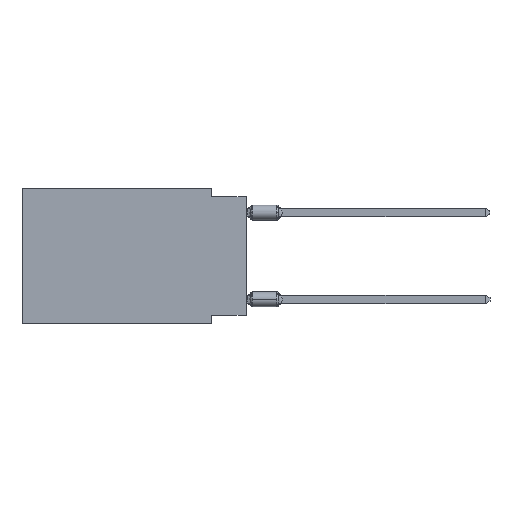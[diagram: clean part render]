
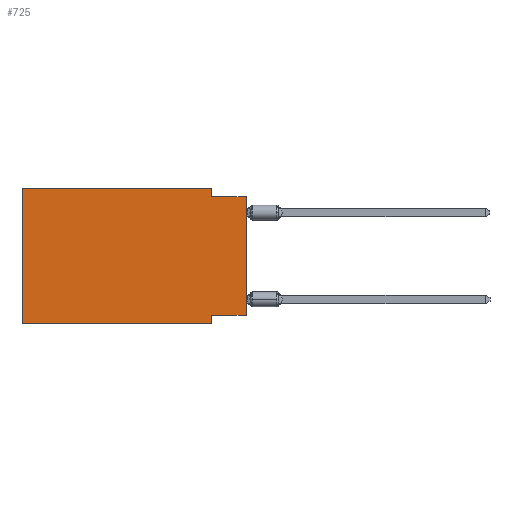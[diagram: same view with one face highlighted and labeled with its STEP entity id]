
A CAD part, left-side view. The second image highlights one B-rep face of the part: STEP entity #725.
In plain terms, the highlighted planar face has unit normal (-1, 0, 0).
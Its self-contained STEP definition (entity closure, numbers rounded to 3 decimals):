
#212 = VERTEX_POINT ( 'NONE', #2073 ) ;
#378 = LINE ( 'NONE', #6083, #16982 ) ;
#499 = CARTESIAN_POINT ( 'NONE',  ( 0., 0., 0. ) ) ;
#627 = DIRECTION ( 'NONE',  ( 0., 0., -1. ) ) ;
#725 = ADVANCED_FACE ( 'NONE', ( #13827 ), #932, .F. ) ;
#876 = LINE ( 'NONE', #6596, #3432 ) ;
#932 = PLANE ( 'NONE',  #6209 ) ;
#1151 = VECTOR ( 'NONE', #627, 1000. ) ;
#1263 = LINE ( 'NONE', #18437, #17861 ) ;
#1679 = VERTEX_POINT ( 'NONE', #16689 ) ;
#1985 = LINE ( 'NONE', #499, #2655 ) ;
#2073 = CARTESIAN_POINT ( 'NONE',  ( 0., 2.54, 0. ) ) ;
#2143 = EDGE_CURVE ( 'NONE', #12360, #1679, #8011, .T. ) ;
#2655 = VECTOR ( 'NONE', #4619, 1000. ) ;
#3432 = VECTOR ( 'NONE', #13870, 1000. ) ;
#3874 = VERTEX_POINT ( 'NONE', #15521 ) ;
#4423 = ORIENTED_EDGE ( 'NONE', *, *, #12769, .F. ) ;
#4619 = DIRECTION ( 'NONE',  ( 0., 0., 1. ) ) ;
#4800 = ORIENTED_EDGE ( 'NONE', *, *, #12511, .F. ) ;
#4975 = ORIENTED_EDGE ( 'NONE', *, *, #7237, .F. ) ;
#5064 = LINE ( 'NONE', #10833, #17888 ) ;
#5314 = DIRECTION ( 'NONE',  ( 1., 0., 0. ) ) ;
#5857 = CARTESIAN_POINT ( 'NONE',  ( 0., 2.54, -0.635 ) ) ;
#6083 = CARTESIAN_POINT ( 'NONE',  ( 0., 0., -9.271 ) ) ;
#6209 = AXIS2_PLACEMENT_3D ( 'NONE', #6644, #5314, #11083 ) ;
#6308 = VECTOR ( 'NONE', #16526, 1000. ) ;
#6451 = LINE ( 'NONE', #17914, #6308 ) ;
#6596 = CARTESIAN_POINT ( 'NONE',  ( 0., 0., -0.635 ) ) ;
#6644 = CARTESIAN_POINT ( 'NONE',  ( 0., 16.383, 0. ) ) ;
#7237 = EDGE_CURVE ( 'NONE', #15447, #7928, #876, .T. ) ;
#7612 = CARTESIAN_POINT ( 'NONE',  ( 0., 2.54, -9.271 ) ) ;
#7653 = ORIENTED_EDGE ( 'NONE', *, *, #2143, .F. ) ;
#7921 = CARTESIAN_POINT ( 'NONE',  ( 0., 2.54, -9.906 ) ) ;
#7928 = VERTEX_POINT ( 'NONE', #15308 ) ;
#8011 = LINE ( 'NONE', #7921, #1151 ) ;
#8789 = EDGE_CURVE ( 'NONE', #3874, #16086, #12790, .T. ) ;
#9051 = ORIENTED_EDGE ( 'NONE', *, *, #11714, .T. ) ;
#9417 = DIRECTION ( 'NONE',  ( 0., 0., -1. ) ) ;
#9775 = CARTESIAN_POINT ( 'NONE',  ( 0., 16.383, 0. ) ) ;
#10750 = VECTOR ( 'NONE', #16990, 1000. ) ;
#10833 = CARTESIAN_POINT ( 'NONE',  ( 0., 2.54, 0. ) ) ;
#11083 = DIRECTION ( 'NONE',  ( 0., 0., -1. ) ) ;
#11714 = EDGE_CURVE ( 'NONE', #3874, #1679, #1263, .T. ) ;
#11810 = ORIENTED_EDGE ( 'NONE', *, *, #14836, .T. ) ;
#11931 = CARTESIAN_POINT ( 'NONE',  ( 0., 0., -9.271 ) ) ;
#12360 = VERTEX_POINT ( 'NONE', #7612 ) ;
#12511 = EDGE_CURVE ( 'NONE', #212, #15447, #5064, .T. ) ;
#12657 = DIRECTION ( 'NONE',  ( 0., -1., 0. ) ) ;
#12727 = VERTEX_POINT ( 'NONE', #11931 ) ;
#12769 = EDGE_CURVE ( 'NONE', #12727, #12360, #378, .T. ) ;
#12790 = LINE ( 'NONE', #9775, #10750 ) ;
#13827 = FACE_OUTER_BOUND ( 'NONE', #16747, .T. ) ;
#13870 = DIRECTION ( 'NONE',  ( 0., -1., 0. ) ) ;
#14836 = EDGE_CURVE ( 'NONE', #12727, #7928, #1985, .T. ) ;
#15247 = CARTESIAN_POINT ( 'NONE',  ( 0., 16.383, 0. ) ) ;
#15308 = CARTESIAN_POINT ( 'NONE',  ( 0., 0., -0.635 ) ) ;
#15447 = VERTEX_POINT ( 'NONE', #5857 ) ;
#15521 = CARTESIAN_POINT ( 'NONE',  ( 0., 16.383, -9.906 ) ) ;
#16086 = VERTEX_POINT ( 'NONE', #15247 ) ;
#16526 = DIRECTION ( 'NONE',  ( 0., -1., 0. ) ) ;
#16689 = CARTESIAN_POINT ( 'NONE',  ( 0., 2.54, -9.906 ) ) ;
#16691 = ORIENTED_EDGE ( 'NONE', *, *, #18228, .F. ) ;
#16747 = EDGE_LOOP ( 'NONE', ( #11810, #4975, #4800, #16691, #16788, #9051, #7653, #4423 ) ) ;
#16788 = ORIENTED_EDGE ( 'NONE', *, *, #8789, .F. ) ;
#16982 = VECTOR ( 'NONE', #17548, 1000. ) ;
#16990 = DIRECTION ( 'NONE',  ( 0., 0., 1. ) ) ;
#17548 = DIRECTION ( 'NONE',  ( 0., 1., 0. ) ) ;
#17861 = VECTOR ( 'NONE', #12657, 1000. ) ;
#17888 = VECTOR ( 'NONE', #9417, 1000. ) ;
#17914 = CARTESIAN_POINT ( 'NONE',  ( 0., 16.383, 0. ) ) ;
#18228 = EDGE_CURVE ( 'NONE', #16086, #212, #6451, .T. ) ;
#18437 = CARTESIAN_POINT ( 'NONE',  ( 0., 16.383, -9.906 ) ) ;
